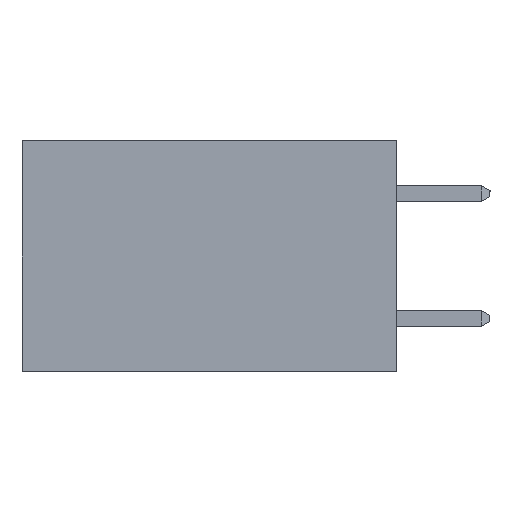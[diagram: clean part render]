
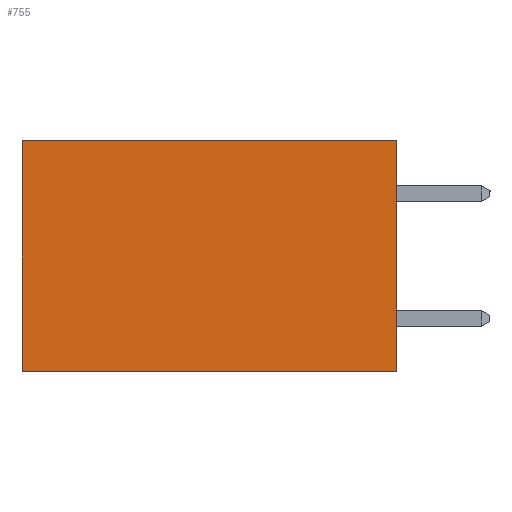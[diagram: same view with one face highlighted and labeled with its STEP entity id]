
A CAD part, left-side view. The second image highlights one B-rep face of the part: STEP entity #755.
In plain terms, the highlighted planar face has unit normal (-1, 0, 0).
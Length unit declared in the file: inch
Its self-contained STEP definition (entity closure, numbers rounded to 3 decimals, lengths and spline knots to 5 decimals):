
#204 = ORIENTED_EDGE ( 'NONE', *, *, #8304, .T. ) ;
#386 = VERTEX_POINT ( 'NONE', #2588 ) ;
#477 = EDGE_CURVE ( 'NONE', #386, #3880, #3267, .T. ) ;
#755 = ADVANCED_FACE ( 'NONE', ( #8575 ), #12576, .F. ) ;
#1643 = VECTOR ( 'NONE', #3840, 39.37008 ) ;
#2323 = CARTESIAN_POINT ( 'NONE',  ( 0.2615, 0., -0.37 ) ) ;
#2588 = CARTESIAN_POINT ( 'NONE',  ( 0.2615, 0., -0.37 ) ) ;
#2619 = ORIENTED_EDGE ( 'NONE', *, *, #477, .F. ) ;
#2661 = CARTESIAN_POINT ( 'NONE',  ( 0.2615, 0., 0. ) ) ;
#2684 = DIRECTION ( 'NONE',  ( 1., 0., 0. ) ) ;
#3133 = CARTESIAN_POINT ( 'NONE',  ( 0.2615, 0., 0. ) ) ;
#3267 = LINE ( 'NONE', #7248, #9869 ) ;
#3308 = VECTOR ( 'NONE', #4385, 39.37008 ) ;
#3393 = EDGE_LOOP ( 'NONE', ( #204, #2619, #9383, #7860 ) ) ;
#3599 = EDGE_CURVE ( 'NONE', #6696, #6299, #10387, .T. ) ;
#3840 = DIRECTION ( 'NONE',  ( 0., 0., -1. ) ) ;
#3880 = VERTEX_POINT ( 'NONE', #7060 ) ;
#4385 = DIRECTION ( 'NONE',  ( 0., 0., -1. ) ) ;
#4878 = EDGE_CURVE ( 'NONE', #6696, #386, #11366, .T. ) ;
#6299 = VERTEX_POINT ( 'NONE', #10051 ) ;
#6630 = DIRECTION ( 'NONE',  ( 0., 0., -1. ) ) ;
#6696 = VERTEX_POINT ( 'NONE', #3133 ) ;
#7060 = CARTESIAN_POINT ( 'NONE',  ( 0.2615, 0.6, -0.37 ) ) ;
#7248 = CARTESIAN_POINT ( 'NONE',  ( 0.2615, 0., -0.37 ) ) ;
#7615 = CARTESIAN_POINT ( 'NONE',  ( 0.2615, 0., -0.37 ) ) ;
#7860 = ORIENTED_EDGE ( 'NONE', *, *, #3599, .T. ) ;
#8304 = EDGE_CURVE ( 'NONE', #6299, #3880, #10689, .T. ) ;
#8575 = FACE_OUTER_BOUND ( 'NONE', #3393, .T. ) ;
#9383 = ORIENTED_EDGE ( 'NONE', *, *, #4878, .F. ) ;
#9640 = CARTESIAN_POINT ( 'NONE',  ( 0.2615, 0.6, -0.37 ) ) ;
#9761 = VECTOR ( 'NONE', #11549, 39.37008 ) ;
#9869 = VECTOR ( 'NONE', #11217, 39.37008 ) ;
#10051 = CARTESIAN_POINT ( 'NONE',  ( 0.2615, 0.6, 0. ) ) ;
#10387 = LINE ( 'NONE', #2661, #9761 ) ;
#10689 = LINE ( 'NONE', #9640, #1643 ) ;
#10915 = AXIS2_PLACEMENT_3D ( 'NONE', #7615, #2684, #6630 ) ;
#11217 = DIRECTION ( 'NONE',  ( 0., 1., 0. ) ) ;
#11366 = LINE ( 'NONE', #2323, #3308 ) ;
#11549 = DIRECTION ( 'NONE',  ( 0., 1., 0. ) ) ;
#12576 = PLANE ( 'NONE',  #10915 ) ;
